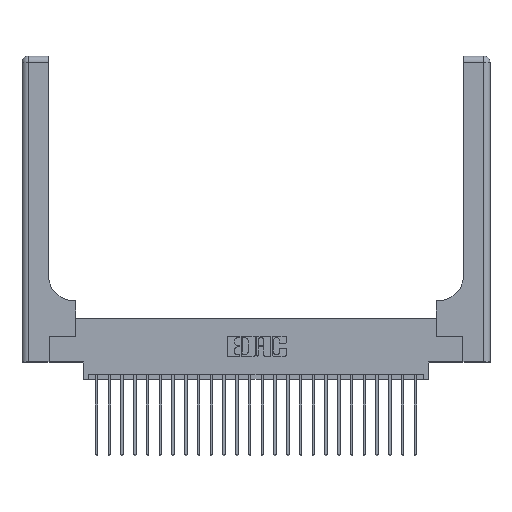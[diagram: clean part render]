
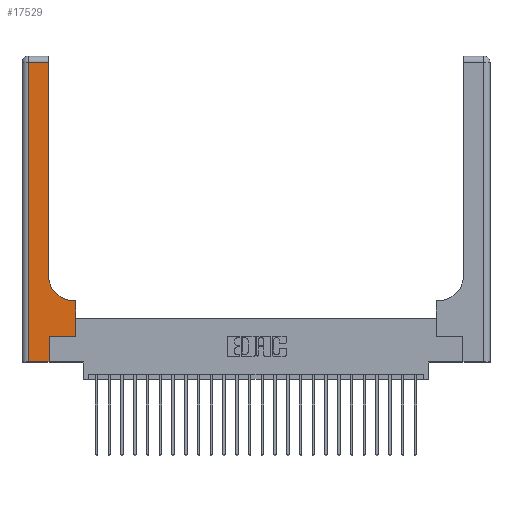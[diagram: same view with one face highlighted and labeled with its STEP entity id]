
A CAD part, top view. The second image highlights one B-rep face of the part: STEP entity #17529.
In plain terms, the highlighted planar face has unit normal (0, 0, 1).
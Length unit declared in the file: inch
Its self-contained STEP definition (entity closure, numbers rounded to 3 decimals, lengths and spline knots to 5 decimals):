
#223 = LINE ( 'NONE', #7619, #19321 ) ;
#531 = DIRECTION ( 'NONE',  ( -1., 0., 0. ) ) ;
#651 = DIRECTION ( 'NONE',  ( 1., 0., 0. ) ) ;
#900 = ORIENTED_EDGE ( 'NONE', *, *, #16153, .T. ) ;
#934 = CARTESIAN_POINT ( 'NONE',  ( 0.26, 0.6, 0.37 ) ) ;
#982 = ORIENTED_EDGE ( 'NONE', *, *, #15350, .T. ) ;
#1012 = CARTESIAN_POINT ( 'NONE',  ( 0.528, 0.25, 0.37 ) ) ;
#1061 = DIRECTION ( 'NONE',  ( -1., 0., 0. ) ) ;
#1071 = ORIENTED_EDGE ( 'NONE', *, *, #7117, .T. ) ;
#1355 = EDGE_CURVE ( 'NONE', #18046, #20945, #11941, .T. ) ;
#1377 = CARTESIAN_POINT ( 'NONE',  ( 0.06, 2.94, 0.37 ) ) ;
#1413 = VERTEX_POINT ( 'NONE', #2779 ) ;
#2779 = CARTESIAN_POINT ( 'NONE',  ( 0.528, 0.6, 0.37 ) ) ;
#3344 = LINE ( 'NONE', #934, #7260 ) ;
#3492 = ORIENTED_EDGE ( 'NONE', *, *, #12494, .T. ) ;
#4102 = VERTEX_POINT ( 'NONE', #9651 ) ;
#4207 = AXIS2_PLACEMENT_3D ( 'NONE', #4385, #17729, #6318 ) ;
#4385 = CARTESIAN_POINT ( 'NONE',  ( 0.51, 0.85, 0.37 ) ) ;
#4833 = ORIENTED_EDGE ( 'NONE', *, *, #18389, .T. ) ;
#4973 = VERTEX_POINT ( 'NONE', #14313 ) ;
#5843 = ORIENTED_EDGE ( 'NONE', *, *, #1355, .T. ) ;
#6318 = DIRECTION ( 'NONE',  ( 1., 0., 0. ) ) ;
#6587 = VECTOR ( 'NONE', #15595, 39.37008 ) ;
#6898 = VECTOR ( 'NONE', #651, 39.37008 ) ;
#7117 = EDGE_CURVE ( 'NONE', #17191, #7821, #21679, .T. ) ;
#7260 = VECTOR ( 'NONE', #21806, 39.37008 ) ;
#7271 = CARTESIAN_POINT ( 'NONE',  ( 0., 0., 0.37 ) ) ;
#7351 = CARTESIAN_POINT ( 'NONE',  ( 0.265, 0., 0.37 ) ) ;
#7619 = CARTESIAN_POINT ( 'NONE',  ( 0.06, 3., 0.37 ) ) ;
#7821 = VERTEX_POINT ( 'NONE', #14109 ) ;
#7942 = ORIENTED_EDGE ( 'NONE', *, *, #22195, .T. ) ;
#8986 = CARTESIAN_POINT ( 'NONE',  ( 0.51, 0.6, 0.37 ) ) ;
#9208 = DIRECTION ( 'NONE',  ( 1., 0., 0. ) ) ;
#9651 = CARTESIAN_POINT ( 'NONE',  ( 0.26, 2.94, 0.37 ) ) ;
#9861 = VECTOR ( 'NONE', #18703, 39.37008 ) ;
#10330 = CARTESIAN_POINT ( 'NONE',  ( 0.265, 0.25, 0.37 ) ) ;
#10370 = DIRECTION ( 'NONE',  ( 0., 1., 0. ) ) ;
#11941 = LINE ( 'NONE', #10330, #6898 ) ;
#12016 = DIRECTION ( 'NONE',  ( 0., 0., -1. ) ) ;
#12494 = EDGE_CURVE ( 'NONE', #22407, #4973, #223, .T. ) ;
#13672 = CARTESIAN_POINT ( 'NONE',  ( 0.528, 0.25, 0.37 ) ) ;
#13944 = ORIENTED_EDGE ( 'NONE', *, *, #22485, .T. ) ;
#14109 = CARTESIAN_POINT ( 'NONE',  ( 0.26, 0.85, 0.37 ) ) ;
#14313 = CARTESIAN_POINT ( 'NONE',  ( 0.06, 0., 0.37 ) ) ;
#14449 = CARTESIAN_POINT ( 'NONE',  ( 0., 2.94, 0.37 ) ) ;
#14497 = LINE ( 'NONE', #7271, #23786 ) ;
#15350 = EDGE_CURVE ( 'NONE', #4102, #22407, #20951, .T. ) ;
#15441 = VECTOR ( 'NONE', #1061, 39.37008 ) ;
#15460 = ORIENTED_EDGE ( 'NONE', *, *, #20651, .T. ) ;
#15595 = DIRECTION ( 'NONE',  ( 0., 1., 0. ) ) ;
#15643 = FACE_OUTER_BOUND ( 'NONE', #23449, .T. ) ;
#16153 = EDGE_CURVE ( 'NONE', #4973, #17811, #14497, .T. ) ;
#17191 = VERTEX_POINT ( 'NONE', #8986 ) ;
#17529 = ADVANCED_FACE ( 'NONE', ( #15643 ), #23212, .F. ) ;
#17729 = DIRECTION ( 'NONE',  ( 0., 0., -1. ) ) ;
#17811 = VERTEX_POINT ( 'NONE', #20299 ) ;
#17930 = LINE ( 'NONE', #13672, #6587 ) ;
#18046 = VERTEX_POINT ( 'NONE', #20857 ) ;
#18149 = LINE ( 'NONE', #7351, #9861 ) ;
#18389 = EDGE_CURVE ( 'NONE', #1413, #17191, #3344, .T. ) ;
#18703 = DIRECTION ( 'NONE',  ( 0., 1., 0. ) ) ;
#19321 = VECTOR ( 'NONE', #22647, 39.37008 ) ;
#19747 = CARTESIAN_POINT ( 'NONE',  ( 0.26, 3., 0.37 ) ) ;
#20299 = CARTESIAN_POINT ( 'NONE',  ( 0.265, 0., 0.37 ) ) ;
#20651 = EDGE_CURVE ( 'NONE', #20945, #1413, #17930, .T. ) ;
#20857 = CARTESIAN_POINT ( 'NONE',  ( 0.265, 0.25, 0.37 ) ) ;
#20945 = VERTEX_POINT ( 'NONE', #1012 ) ;
#20951 = LINE ( 'NONE', #14449, #15441 ) ;
#21269 = CARTESIAN_POINT ( 'NONE',  ( 0., 3., 0.37 ) ) ;
#21679 = CIRCLE ( 'NONE', #4207, 0.25 ) ;
#21806 = DIRECTION ( 'NONE',  ( -1., 0., 0. ) ) ;
#22195 = EDGE_CURVE ( 'NONE', #7821, #4102, #23311, .T. ) ;
#22407 = VERTEX_POINT ( 'NONE', #1377 ) ;
#22485 = EDGE_CURVE ( 'NONE', #17811, #18046, #18149, .T. ) ;
#22531 = AXIS2_PLACEMENT_3D ( 'NONE', #21269, #12016, #531 ) ;
#22647 = DIRECTION ( 'NONE',  ( 0., -1., 0. ) ) ;
#23212 = PLANE ( 'NONE',  #22531 ) ;
#23311 = LINE ( 'NONE', #19747, #23874 ) ;
#23449 = EDGE_LOOP ( 'NONE', ( #7942, #982, #3492, #900, #13944, #5843, #15460, #4833, #1071 ) ) ;
#23786 = VECTOR ( 'NONE', #9208, 39.37008 ) ;
#23874 = VECTOR ( 'NONE', #10370, 39.37008 ) ;
